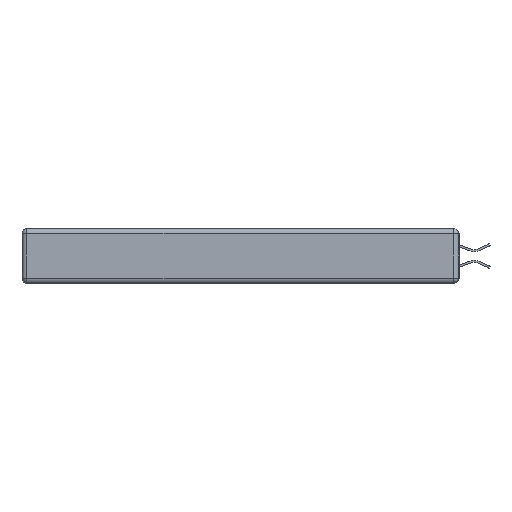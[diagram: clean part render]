
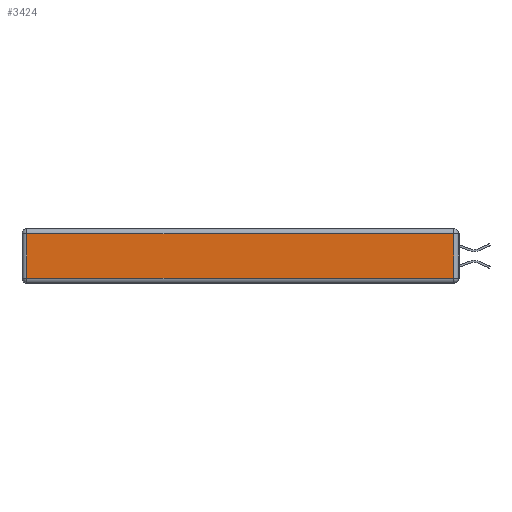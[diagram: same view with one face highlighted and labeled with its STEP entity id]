
A CAD part, left-side view. The second image highlights one B-rep face of the part: STEP entity #3424.
In plain terms, the highlighted planar face has unit normal (-1, 0, 0).
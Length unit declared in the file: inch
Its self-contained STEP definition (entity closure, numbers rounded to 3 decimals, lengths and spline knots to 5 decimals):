
#21 = EDGE_CURVE ( 'NONE', #1768, #11128, #3325, .T. ) ;
#756 = VECTOR ( 'NONE', #8987, 39.37008 ) ;
#1341 = DIRECTION ( 'NONE',  ( 0., 0., 1. ) ) ;
#1548 = VECTOR ( 'NONE', #1998, 39.37008 ) ;
#1768 = VERTEX_POINT ( 'NONE', #2125 ) ;
#1998 = DIRECTION ( 'NONE',  ( 0., 0., 1. ) ) ;
#2125 = CARTESIAN_POINT ( 'NONE',  ( 0., 0.03, -0.03 ) ) ;
#3147 = VECTOR ( 'NONE', #5830, 39.37008 ) ;
#3325 = LINE ( 'NONE', #14721, #11095 ) ;
#3347 = EDGE_CURVE ( 'NONE', #9165, #4231, #8832, .T. ) ;
#3424 = ADVANCED_FACE ( 'NONE', ( #9009 ), #13895, .T. ) ;
#3818 = CARTESIAN_POINT ( 'NONE',  ( 0., 0.03, -0.343 ) ) ;
#4231 = VERTEX_POINT ( 'NONE', #10635 ) ;
#4391 = CARTESIAN_POINT ( 'NONE',  ( 0., 0., -0.313 ) ) ;
#4855 = CARTESIAN_POINT ( 'NONE',  ( 0., 2.72, -0.03 ) ) ;
#5830 = DIRECTION ( 'NONE',  ( 0., 0., -1. ) ) ;
#6432 = ORIENTED_EDGE ( 'NONE', *, *, #3347, .T. ) ;
#7011 = DIRECTION ( 'NONE',  ( -1., 0., 0. ) ) ;
#7124 = EDGE_CURVE ( 'NONE', #11128, #9165, #9275, .T. ) ;
#7140 = ORIENTED_EDGE ( 'NONE', *, *, #7124, .T. ) ;
#8045 = CARTESIAN_POINT ( 'NONE',  ( 0., 2.72, -0.343 ) ) ;
#8149 = EDGE_LOOP ( 'NONE', ( #6432, #14616, #12186, #7140 ) ) ;
#8612 = CARTESIAN_POINT ( 'NONE',  ( 0., 2.72, -0.313 ) ) ;
#8832 = LINE ( 'NONE', #4391, #756 ) ;
#8987 = DIRECTION ( 'NONE',  ( 0., -1., 0. ) ) ;
#9009 = FACE_OUTER_BOUND ( 'NONE', #8149, .T. ) ;
#9165 = VERTEX_POINT ( 'NONE', #8612 ) ;
#9275 = LINE ( 'NONE', #8045, #3147 ) ;
#10017 = LINE ( 'NONE', #3818, #1548 ) ;
#10404 = CARTESIAN_POINT ( 'NONE',  ( 0., 0., -0.343 ) ) ;
#10635 = CARTESIAN_POINT ( 'NONE',  ( 0., 0.03, -0.313 ) ) ;
#11095 = VECTOR ( 'NONE', #12496, 39.37008 ) ;
#11128 = VERTEX_POINT ( 'NONE', #4855 ) ;
#11186 = EDGE_CURVE ( 'NONE', #4231, #1768, #10017, .T. ) ;
#12186 = ORIENTED_EDGE ( 'NONE', *, *, #21, .T. ) ;
#12496 = DIRECTION ( 'NONE',  ( 0., 1., 0. ) ) ;
#13895 = PLANE ( 'NONE',  #14826 ) ;
#14616 = ORIENTED_EDGE ( 'NONE', *, *, #11186, .T. ) ;
#14721 = CARTESIAN_POINT ( 'NONE',  ( 0., 2.75, -0.03 ) ) ;
#14826 = AXIS2_PLACEMENT_3D ( 'NONE', #10404, #7011, #1341 ) ;
